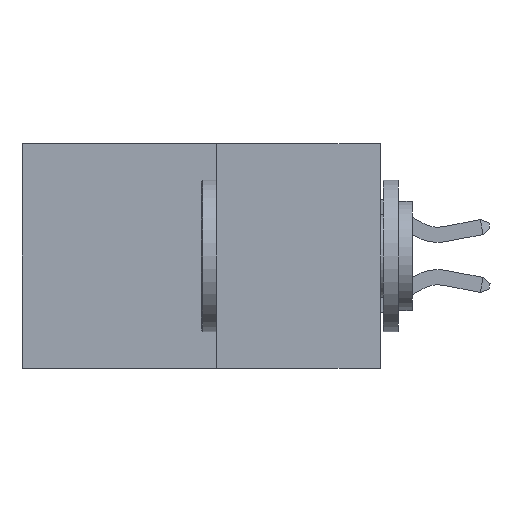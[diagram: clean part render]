
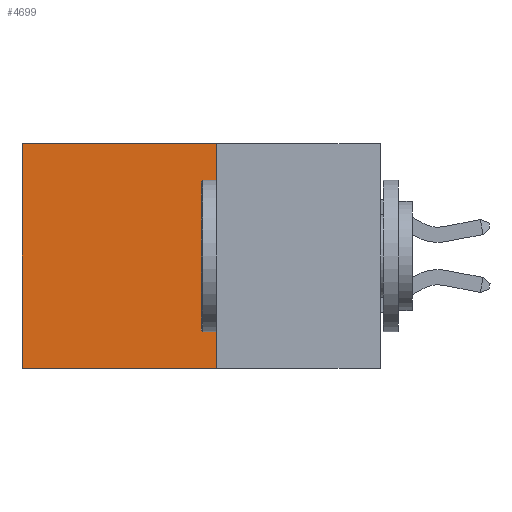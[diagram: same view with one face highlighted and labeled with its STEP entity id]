
A CAD part, left-side view. The second image highlights one B-rep face of the part: STEP entity #4699.
In plain terms, the highlighted planar face has unit normal (-1, 0, 0).
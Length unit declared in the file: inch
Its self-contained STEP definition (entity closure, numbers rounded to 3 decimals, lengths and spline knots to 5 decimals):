
#145 = CARTESIAN_POINT ( 'NONE',  ( 0.277, 0.27, -0.37 ) ) ;
#286 = CARTESIAN_POINT ( 'NONE',  ( 0.277, 0.27, -0.37 ) ) ;
#728 = VERTEX_POINT ( 'NONE', #286 ) ;
#744 = CARTESIAN_POINT ( 'NONE',  ( 0.277, 0.59, 0. ) ) ;
#1020 = DIRECTION ( 'NONE',  ( 0., 0., -1. ) ) ;
#1027 = DIRECTION ( 'NONE',  ( 1., 0., 0. ) ) ;
#1152 = PLANE ( 'NONE',  #7981 ) ;
#1165 = CARTESIAN_POINT ( 'NONE',  ( 0.277, 0.27, -0.37 ) ) ;
#1239 = LINE ( 'NONE', #9895, #7579 ) ;
#1322 = LINE ( 'NONE', #6601, #9483 ) ;
#1346 = ORIENTED_EDGE ( 'NONE', *, *, #3936, .F. ) ;
#1474 = LINE ( 'NONE', #145, #9629 ) ;
#1914 = FACE_OUTER_BOUND ( 'NONE', #2608, .T. ) ;
#1965 = EDGE_CURVE ( 'NONE', #2768, #6602, #4248, .T. ) ;
#2150 = VECTOR ( 'NONE', #6561, 39.37008 ) ;
#2608 = EDGE_LOOP ( 'NONE', ( #9278, #1346, #7695, #9755 ) ) ;
#2768 = VERTEX_POINT ( 'NONE', #5318 ) ;
#3165 = VERTEX_POINT ( 'NONE', #9743 ) ;
#3936 = EDGE_CURVE ( 'NONE', #728, #3165, #1322, .T. ) ;
#4248 = LINE ( 'NONE', #7540, #2150 ) ;
#4699 = ADVANCED_FACE ( 'NONE', ( #1914 ), #1152, .F. ) ;
#5188 = DIRECTION ( 'NONE',  ( 0., 0., -1. ) ) ;
#5318 = CARTESIAN_POINT ( 'NONE',  ( 0.277, 0.27, 0. ) ) ;
#6559 = DIRECTION ( 'NONE',  ( 0., 0., -1. ) ) ;
#6561 = DIRECTION ( 'NONE',  ( 0., 1., 0. ) ) ;
#6601 = CARTESIAN_POINT ( 'NONE',  ( 0.277, 0.27, -0.37 ) ) ;
#6602 = VERTEX_POINT ( 'NONE', #744 ) ;
#7540 = CARTESIAN_POINT ( 'NONE',  ( 0.277, 0.27, 0. ) ) ;
#7579 = VECTOR ( 'NONE', #5188, 39.37008 ) ;
#7695 = ORIENTED_EDGE ( 'NONE', *, *, #9654, .F. ) ;
#7981 = AXIS2_PLACEMENT_3D ( 'NONE', #1165, #1027, #1020 ) ;
#8490 = EDGE_CURVE ( 'NONE', #6602, #3165, #1239, .T. ) ;
#9278 = ORIENTED_EDGE ( 'NONE', *, *, #8490, .T. ) ;
#9483 = VECTOR ( 'NONE', #9785, 39.37008 ) ;
#9629 = VECTOR ( 'NONE', #6559, 39.37008 ) ;
#9654 = EDGE_CURVE ( 'NONE', #2768, #728, #1474, .T. ) ;
#9743 = CARTESIAN_POINT ( 'NONE',  ( 0.277, 0.59, -0.37 ) ) ;
#9755 = ORIENTED_EDGE ( 'NONE', *, *, #1965, .T. ) ;
#9785 = DIRECTION ( 'NONE',  ( 0., 1., 0. ) ) ;
#9895 = CARTESIAN_POINT ( 'NONE',  ( 0.277, 0.59, -0.37 ) ) ;
